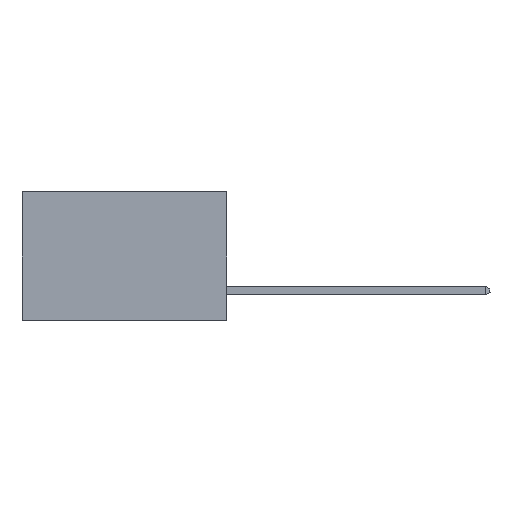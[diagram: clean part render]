
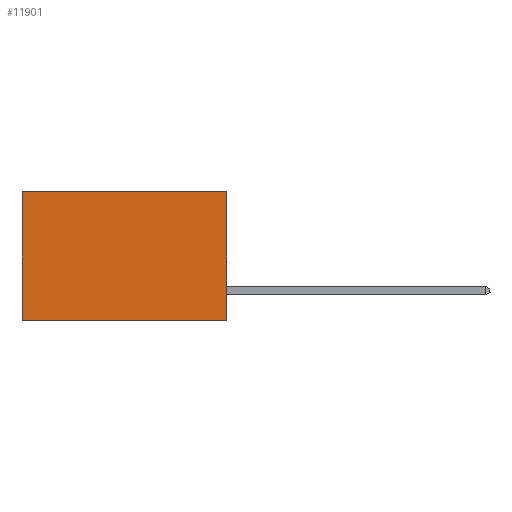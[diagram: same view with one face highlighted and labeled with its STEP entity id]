
A CAD part, left-side view. The second image highlights one B-rep face of the part: STEP entity #11901.
In plain terms, the highlighted planar face has unit normal (-1, 0, 0).
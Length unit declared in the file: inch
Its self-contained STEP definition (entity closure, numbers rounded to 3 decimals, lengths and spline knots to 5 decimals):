
#143 = VECTOR ( 'NONE', #6385, 39.37008 ) ;
#218 = EDGE_CURVE ( 'NONE', #7543, #16516, #4723, .T. ) ;
#257 = EDGE_CURVE ( 'NONE', #4001, #7543, #4257, .T. ) ;
#969 = VECTOR ( 'NONE', #8969, 39.37008 ) ;
#1296 = CARTESIAN_POINT ( 'NONE',  ( 0.277, 0.59, 0. ) ) ;
#1799 = ORIENTED_EDGE ( 'NONE', *, *, #257, .F. ) ;
#2177 = AXIS2_PLACEMENT_3D ( 'NONE', #16736, #2421, #11744 ) ;
#2258 = ORIENTED_EDGE ( 'NONE', *, *, #3604, .T. ) ;
#2421 = DIRECTION ( 'NONE',  ( 1., 0., 0. ) ) ;
#3133 = EDGE_CURVE ( 'NONE', #12751, #16516, #3924, .T. ) ;
#3604 = EDGE_CURVE ( 'NONE', #4001, #12751, #13771, .T. ) ;
#3924 = LINE ( 'NONE', #6611, #143 ) ;
#4001 = VERTEX_POINT ( 'NONE', #7373 ) ;
#4257 = LINE ( 'NONE', #5595, #13488 ) ;
#4723 = LINE ( 'NONE', #11665, #969 ) ;
#5595 = CARTESIAN_POINT ( 'NONE',  ( 0.277, 0., -0.37 ) ) ;
#6385 = DIRECTION ( 'NONE',  ( 0., 0., -1. ) ) ;
#6440 = FACE_OUTER_BOUND ( 'NONE', #8533, .T. ) ;
#6611 = CARTESIAN_POINT ( 'NONE',  ( 0.277, 0.59, -0.37 ) ) ;
#7277 = VECTOR ( 'NONE', #12896, 39.37008 ) ;
#7373 = CARTESIAN_POINT ( 'NONE',  ( 0.277, 0., 0. ) ) ;
#7543 = VERTEX_POINT ( 'NONE', #7810 ) ;
#7810 = CARTESIAN_POINT ( 'NONE',  ( 0.277, 0., -0.37 ) ) ;
#8533 = EDGE_LOOP ( 'NONE', ( #12062, #15476, #1799, #2258 ) ) ;
#8969 = DIRECTION ( 'NONE',  ( 0., 1., 0. ) ) ;
#9569 = CARTESIAN_POINT ( 'NONE',  ( 0.277, 0.59, -0.37 ) ) ;
#10426 = PLANE ( 'NONE',  #2177 ) ;
#10593 = DIRECTION ( 'NONE',  ( 0., 0., -1. ) ) ;
#11665 = CARTESIAN_POINT ( 'NONE',  ( 0.277, 0., -0.37 ) ) ;
#11744 = DIRECTION ( 'NONE',  ( 0., 0., -1. ) ) ;
#11901 = ADVANCED_FACE ( 'NONE', ( #6440 ), #10426, .F. ) ;
#12062 = ORIENTED_EDGE ( 'NONE', *, *, #3133, .T. ) ;
#12751 = VERTEX_POINT ( 'NONE', #1296 ) ;
#12896 = DIRECTION ( 'NONE',  ( 0., 1., 0. ) ) ;
#13488 = VECTOR ( 'NONE', #10593, 39.37008 ) ;
#13771 = LINE ( 'NONE', #16592, #7277 ) ;
#15476 = ORIENTED_EDGE ( 'NONE', *, *, #218, .F. ) ;
#16516 = VERTEX_POINT ( 'NONE', #9569 ) ;
#16592 = CARTESIAN_POINT ( 'NONE',  ( 0.277, 0., 0. ) ) ;
#16736 = CARTESIAN_POINT ( 'NONE',  ( 0.277, 0., -0.37 ) ) ;
